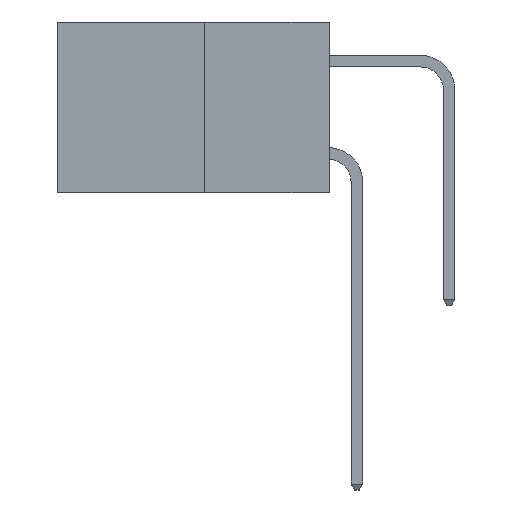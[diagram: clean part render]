
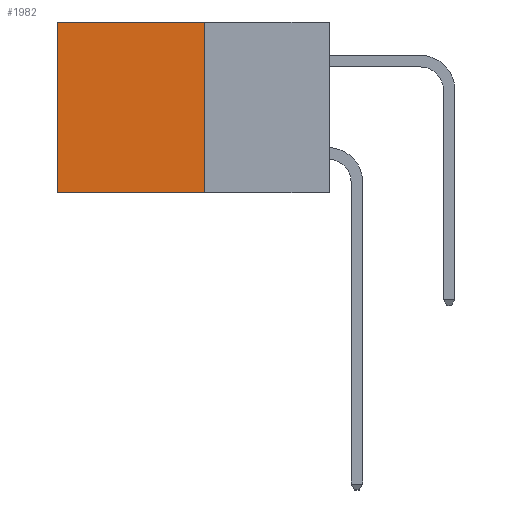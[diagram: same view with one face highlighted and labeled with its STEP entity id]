
A CAD part, left-side view. The second image highlights one B-rep face of the part: STEP entity #1982.
In plain terms, the highlighted planar face has unit normal (-1, 0, 0).
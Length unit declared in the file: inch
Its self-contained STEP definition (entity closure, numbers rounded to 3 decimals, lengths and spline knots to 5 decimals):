
#625 = VECTOR ( 'NONE', #9617, 39.37008 ) ;
#640 = LINE ( 'NONE', #5593, #4923 ) ;
#958 = VERTEX_POINT ( 'NONE', #8806 ) ;
#1982 = ADVANCED_FACE ( 'NONE', ( #7055 ), #5406, .F. ) ;
#2563 = DIRECTION ( 'NONE',  ( 0., 1., 0. ) ) ;
#2667 = ORIENTED_EDGE ( 'NONE', *, *, #7807, .T. ) ;
#2732 = CARTESIAN_POINT ( 'NONE',  ( 0.277, 0.27, 0. ) ) ;
#2769 = DIRECTION ( 'NONE',  ( 1., 0., 0. ) ) ;
#3154 = DIRECTION ( 'NONE',  ( 0., 0., -1. ) ) ;
#3268 = CARTESIAN_POINT ( 'NONE',  ( 0.277, 0.59, -0.37 ) ) ;
#4660 = AXIS2_PLACEMENT_3D ( 'NONE', #5631, #2769, #8696 ) ;
#4923 = VECTOR ( 'NONE', #5502, 39.37008 ) ;
#5162 = LINE ( 'NONE', #5970, #625 ) ;
#5292 = VECTOR ( 'NONE', #2563, 39.37008 ) ;
#5406 = PLANE ( 'NONE',  #4660 ) ;
#5502 = DIRECTION ( 'NONE',  ( 0., 0., -1. ) ) ;
#5593 = CARTESIAN_POINT ( 'NONE',  ( 0.277, 0.27, -0.37 ) ) ;
#5631 = CARTESIAN_POINT ( 'NONE',  ( 0.277, 0.27, -0.37 ) ) ;
#5970 = CARTESIAN_POINT ( 'NONE',  ( 0.277, 0.27, -0.37 ) ) ;
#6628 = VERTEX_POINT ( 'NONE', #8498 ) ;
#6764 = CARTESIAN_POINT ( 'NONE',  ( 0.277, 0.59, -0.37 ) ) ;
#6836 = ORIENTED_EDGE ( 'NONE', *, *, #8136, .F. ) ;
#6909 = VERTEX_POINT ( 'NONE', #6764 ) ;
#7055 = FACE_OUTER_BOUND ( 'NONE', #9762, .T. ) ;
#7279 = LINE ( 'NONE', #2732, #5292 ) ;
#7590 = EDGE_CURVE ( 'NONE', #6628, #8519, #640, .T. ) ;
#7606 = ORIENTED_EDGE ( 'NONE', *, *, #7782, .T. ) ;
#7782 = EDGE_CURVE ( 'NONE', #958, #6909, #7958, .T. ) ;
#7807 = EDGE_CURVE ( 'NONE', #6628, #958, #7279, .T. ) ;
#7958 = LINE ( 'NONE', #3268, #9441 ) ;
#8136 = EDGE_CURVE ( 'NONE', #8519, #6909, #5162, .T. ) ;
#8498 = CARTESIAN_POINT ( 'NONE',  ( 0.277, 0.27, 0. ) ) ;
#8519 = VERTEX_POINT ( 'NONE', #9405 ) ;
#8696 = DIRECTION ( 'NONE',  ( 0., 0., -1. ) ) ;
#8806 = CARTESIAN_POINT ( 'NONE',  ( 0.277, 0.59, 0. ) ) ;
#8884 = ORIENTED_EDGE ( 'NONE', *, *, #7590, .F. ) ;
#9405 = CARTESIAN_POINT ( 'NONE',  ( 0.277, 0.27, -0.37 ) ) ;
#9441 = VECTOR ( 'NONE', #3154, 39.37008 ) ;
#9617 = DIRECTION ( 'NONE',  ( 0., 1., 0. ) ) ;
#9762 = EDGE_LOOP ( 'NONE', ( #7606, #6836, #8884, #2667 ) ) ;
